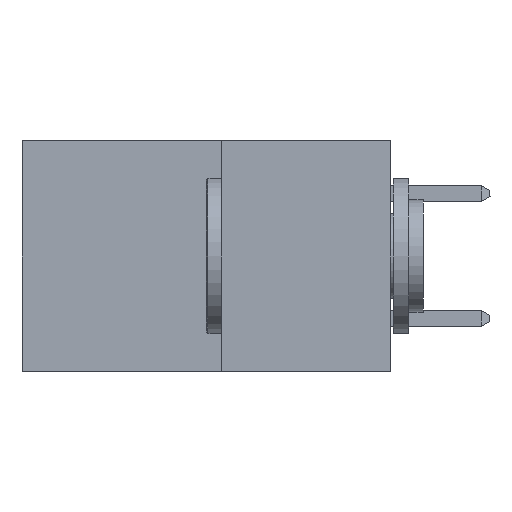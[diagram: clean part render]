
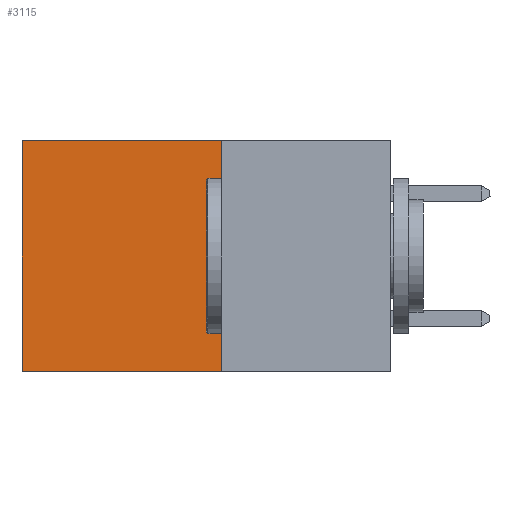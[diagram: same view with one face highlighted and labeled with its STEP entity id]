
A CAD part, left-side view. The second image highlights one B-rep face of the part: STEP entity #3115.
In plain terms, the highlighted planar face has unit normal (-1, 0, 0).
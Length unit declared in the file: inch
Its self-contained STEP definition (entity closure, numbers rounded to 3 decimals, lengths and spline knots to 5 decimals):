
#2296 = VECTOR ( 'NONE', #10506, 39.37008 ) ;
#3115 = ADVANCED_FACE ( 'NONE', ( #25362 ), #17978, .F. ) ;
#5343 = CARTESIAN_POINT ( 'NONE',  ( 0.277, 0.59, 0. ) ) ;
#6225 = EDGE_CURVE ( 'NONE', #6496, #25006, #30017, .T. ) ;
#6426 = CARTESIAN_POINT ( 'NONE',  ( 0.277, 0.27, 0. ) ) ;
#6496 = VERTEX_POINT ( 'NONE', #6426 ) ;
#6899 = EDGE_CURVE ( 'NONE', #31782, #32166, #31656, .T. ) ;
#6958 = CARTESIAN_POINT ( 'NONE',  ( 0.277, 0.59, -0.37 ) ) ;
#7979 = CARTESIAN_POINT ( 'NONE',  ( 0.277, 0.27, 0. ) ) ;
#9305 = LINE ( 'NONE', #31190, #2296 ) ;
#9554 = VECTOR ( 'NONE', #10576, 39.37008 ) ;
#10506 = DIRECTION ( 'NONE',  ( 0., 1., 0. ) ) ;
#10576 = DIRECTION ( 'NONE',  ( 0., 1., 0. ) ) ;
#10907 = VECTOR ( 'NONE', #30973, 39.37008 ) ;
#12818 = LINE ( 'NONE', #7979, #9554 ) ;
#17360 = DIRECTION ( 'NONE',  ( 0., 0., -1. ) ) ;
#17675 = ORIENTED_EDGE ( 'NONE', *, *, #6899, .T. ) ;
#17678 = DIRECTION ( 'NONE',  ( 1., 0., 0. ) ) ;
#17978 = PLANE ( 'NONE',  #27623 ) ;
#18113 = EDGE_CURVE ( 'NONE', #25006, #32166, #9305, .T. ) ;
#18674 = CARTESIAN_POINT ( 'NONE',  ( 0.277, 0.27, -0.37 ) ) ;
#20627 = ORIENTED_EDGE ( 'NONE', *, *, #18113, .F. ) ;
#21768 = ORIENTED_EDGE ( 'NONE', *, *, #6225, .F. ) ;
#22120 = CARTESIAN_POINT ( 'NONE',  ( 0.277, 0.27, -0.37 ) ) ;
#22608 = DIRECTION ( 'NONE',  ( 0., 0., -1. ) ) ;
#22890 = CARTESIAN_POINT ( 'NONE',  ( 0.277, 0.27, -0.37 ) ) ;
#23077 = VECTOR ( 'NONE', #22608, 39.37008 ) ;
#25006 = VERTEX_POINT ( 'NONE', #22120 ) ;
#25362 = FACE_OUTER_BOUND ( 'NONE', #27671, .T. ) ;
#25967 = EDGE_CURVE ( 'NONE', #6496, #31782, #12818, .T. ) ;
#26542 = ORIENTED_EDGE ( 'NONE', *, *, #25967, .T. ) ;
#27623 = AXIS2_PLACEMENT_3D ( 'NONE', #18674, #17678, #17360 ) ;
#27671 = EDGE_LOOP ( 'NONE', ( #17675, #20627, #21768, #26542 ) ) ;
#30017 = LINE ( 'NONE', #22890, #23077 ) ;
#30973 = DIRECTION ( 'NONE',  ( 0., 0., -1. ) ) ;
#31190 = CARTESIAN_POINT ( 'NONE',  ( 0.277, 0.27, -0.37 ) ) ;
#31315 = CARTESIAN_POINT ( 'NONE',  ( 0.277, 0.59, -0.37 ) ) ;
#31656 = LINE ( 'NONE', #31315, #10907 ) ;
#31782 = VERTEX_POINT ( 'NONE', #5343 ) ;
#32166 = VERTEX_POINT ( 'NONE', #6958 ) ;
